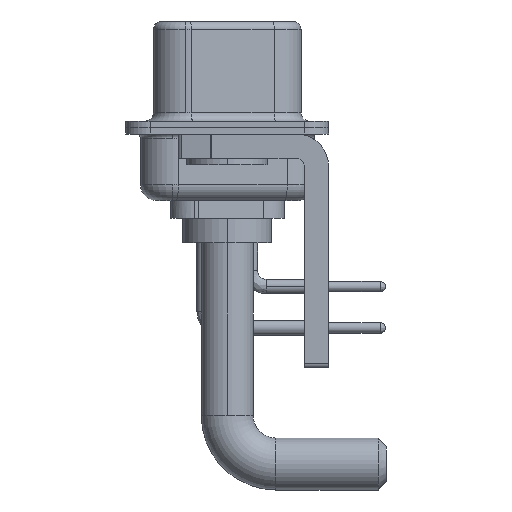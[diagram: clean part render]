
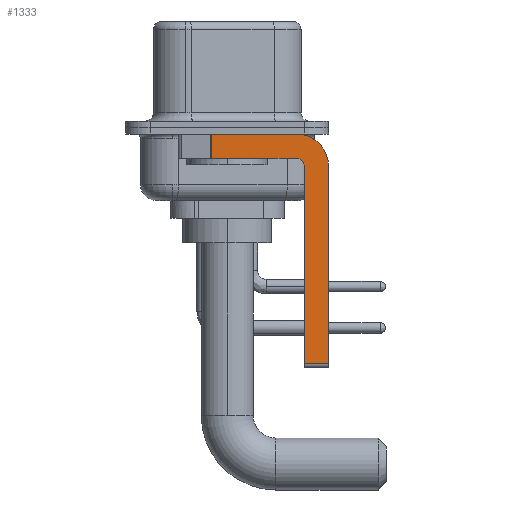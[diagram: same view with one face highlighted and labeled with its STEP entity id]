
A CAD part, left-side view. The second image highlights one B-rep face of the part: STEP entity #1333.
In plain terms, the highlighted planar face has unit normal (-1, 0, 0).
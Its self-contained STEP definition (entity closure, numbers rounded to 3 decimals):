
#12 = CARTESIAN_POINT ( 'NONE',  ( -2.9, -4.25, -0.4 ) ) ;
#357 = CARTESIAN_POINT ( 'NONE',  ( -2.9, -4.25, -1.9 ) ) ;
#428 = LINE ( 'NONE', #16723, #16990 ) ;
#1233 = AXIS2_PLACEMENT_3D ( 'NONE', #6077, #25725, #3986 ) ;
#1333 = ADVANCED_FACE ( 'NONE', ( #14834 ), #25170, .F. ) ;
#1352 = VECTOR ( 'NONE', #16948, 1000. ) ;
#1379 = VECTOR ( 'NONE', #21694, 1000. ) ;
#1677 = AXIS2_PLACEMENT_3D ( 'NONE', #17181, #9078, #2684 ) ;
#1727 = DIRECTION ( 'NONE',  ( 0., 0., 1. ) ) ;
#1859 = LINE ( 'NONE', #5890, #23429 ) ;
#2559 = CIRCLE ( 'NONE', #1677, 2. ) ;
#2684 = DIRECTION ( 'NONE',  ( 0., 0., -1. ) ) ;
#2694 = AXIS2_PLACEMENT_3D ( 'NONE', #4331, #8487, #25500 ) ;
#3415 = EDGE_LOOP ( 'NONE', ( #26525, #23763, #7423, #11309, #6248, #14968, #9163, #19868 ) ) ;
#3448 = VERTEX_POINT ( 'NONE', #6168 ) ;
#3936 = DIRECTION ( 'NONE',  ( 0., 1., 0. ) ) ;
#3986 = DIRECTION ( 'NONE',  ( 0., 0., -1. ) ) ;
#4331 = CARTESIAN_POINT ( 'NONE',  ( -2.9, -4.25, -2.4 ) ) ;
#5049 = CARTESIAN_POINT ( 'NONE',  ( -2.9, -6.25, -2.4 ) ) ;
#5890 = CARTESIAN_POINT ( 'NONE',  ( -2.9, -4.75, -14.8 ) ) ;
#6077 = CARTESIAN_POINT ( 'NONE',  ( -2.9, -4.25, -2.4 ) ) ;
#6168 = CARTESIAN_POINT ( 'NONE',  ( -2.9, -6.25, -14.55 ) ) ;
#6248 = ORIENTED_EDGE ( 'NONE', *, *, #6458, .F. ) ;
#6458 = EDGE_CURVE ( 'NONE', #20175, #12838, #1859, .T. ) ;
#6804 = EDGE_CURVE ( 'NONE', #19096, #12988, #8083, .T. ) ;
#7008 = EDGE_CURVE ( 'NONE', #20218, #17816, #2559, .T. ) ;
#7423 = ORIENTED_EDGE ( 'NONE', *, *, #6804, .F. ) ;
#7779 = DIRECTION ( 'NONE',  ( 0., 0., -1. ) ) ;
#8083 = LINE ( 'NONE', #23135, #25673 ) ;
#8212 = CARTESIAN_POINT ( 'NONE',  ( -2.9, -4.75, -14.55 ) ) ;
#8487 = DIRECTION ( 'NONE',  ( -1., 0., 0. ) ) ;
#8593 = LINE ( 'NONE', #16819, #1352 ) ;
#9078 = DIRECTION ( 'NONE',  ( 1., 0., 0. ) ) ;
#9163 = ORIENTED_EDGE ( 'NONE', *, *, #11244, .F. ) ;
#9338 = CIRCLE ( 'NONE', #2694, 0.5 ) ;
#10865 = DIRECTION ( 'NONE',  ( 0., -1., 0. ) ) ;
#11244 = EDGE_CURVE ( 'NONE', #17816, #3448, #18352, .T. ) ;
#11309 = ORIENTED_EDGE ( 'NONE', *, *, #25797, .F. ) ;
#12838 = VERTEX_POINT ( 'NONE', #16433 ) ;
#12988 = VERTEX_POINT ( 'NONE', #22980 ) ;
#14834 = FACE_OUTER_BOUND ( 'NONE', #3415, .T. ) ;
#14855 = EDGE_CURVE ( 'NONE', #16414, #20218, #21144, .T. ) ;
#14920 = EDGE_CURVE ( 'NONE', #16414, #12988, #8593, .T. ) ;
#14968 = ORIENTED_EDGE ( 'NONE', *, *, #26931, .T. ) ;
#16414 = VERTEX_POINT ( 'NONE', #21138 ) ;
#16433 = CARTESIAN_POINT ( 'NONE',  ( -2.9, -4.75, -2.4 ) ) ;
#16723 = CARTESIAN_POINT ( 'NONE',  ( -2.9, -4.25, -14.55 ) ) ;
#16819 = CARTESIAN_POINT ( 'NONE',  ( -2.9, 0.978, -1.9 ) ) ;
#16948 = DIRECTION ( 'NONE',  ( 0., 0., -1. ) ) ;
#16990 = VECTOR ( 'NONE', #10865, 1000. ) ;
#17181 = CARTESIAN_POINT ( 'NONE',  ( -2.9, -4.25, -2.4 ) ) ;
#17816 = VERTEX_POINT ( 'NONE', #5049 ) ;
#18352 = LINE ( 'NONE', #26869, #18432 ) ;
#18432 = VECTOR ( 'NONE', #7779, 1000. ) ;
#19096 = VERTEX_POINT ( 'NONE', #357 ) ;
#19868 = ORIENTED_EDGE ( 'NONE', *, *, #7008, .F. ) ;
#20175 = VERTEX_POINT ( 'NONE', #8212 ) ;
#20218 = VERTEX_POINT ( 'NONE', #12 ) ;
#21138 = CARTESIAN_POINT ( 'NONE',  ( -2.9, 0.978, -0.4 ) ) ;
#21144 = LINE ( 'NONE', #25749, #1379 ) ;
#21694 = DIRECTION ( 'NONE',  ( 0., -1., 0. ) ) ;
#22980 = CARTESIAN_POINT ( 'NONE',  ( -2.9, 0.978, -1.9 ) ) ;
#23135 = CARTESIAN_POINT ( 'NONE',  ( -2.9, -4.25, -1.9 ) ) ;
#23429 = VECTOR ( 'NONE', #1727, 1000. ) ;
#23763 = ORIENTED_EDGE ( 'NONE', *, *, #14920, .T. ) ;
#25170 = PLANE ( 'NONE',  #1233 ) ;
#25500 = DIRECTION ( 'NONE',  ( 0., 0., 1. ) ) ;
#25673 = VECTOR ( 'NONE', #3936, 1000. ) ;
#25725 = DIRECTION ( 'NONE',  ( 1., 0., 0. ) ) ;
#25749 = CARTESIAN_POINT ( 'NONE',  ( -2.9, 3., -0.4 ) ) ;
#25797 = EDGE_CURVE ( 'NONE', #12838, #19096, #9338, .T. ) ;
#26525 = ORIENTED_EDGE ( 'NONE', *, *, #14855, .F. ) ;
#26869 = CARTESIAN_POINT ( 'NONE',  ( -2.9, -6.25, -2.4 ) ) ;
#26931 = EDGE_CURVE ( 'NONE', #20175, #3448, #428, .T. ) ;
